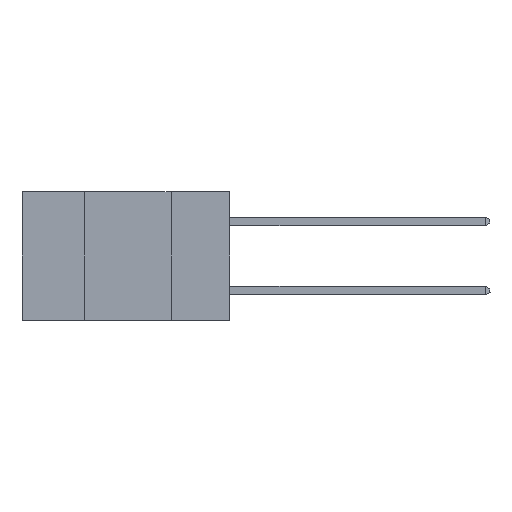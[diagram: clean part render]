
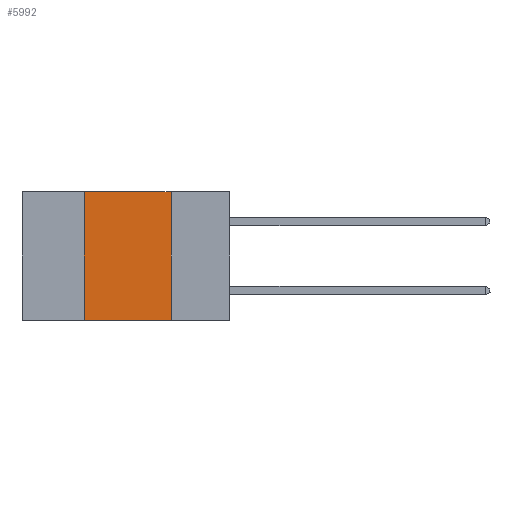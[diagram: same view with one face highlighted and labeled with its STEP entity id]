
A CAD part, left-side view. The second image highlights one B-rep face of the part: STEP entity #5992.
In plain terms, the highlighted planar face has unit normal (-1, 0, 0).
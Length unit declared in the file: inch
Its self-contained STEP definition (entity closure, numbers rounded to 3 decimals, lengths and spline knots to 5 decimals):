
#988 = CARTESIAN_POINT ( 'NONE',  ( 0., 0.6, 0. ) ) ;
#1178 = VERTEX_POINT ( 'NONE', #13964 ) ;
#1229 = VERTEX_POINT ( 'NONE', #21943 ) ;
#1454 = VERTEX_POINT ( 'NONE', #7531 ) ;
#2304 = VERTEX_POINT ( 'NONE', #19432 ) ;
#2470 = ORIENTED_EDGE ( 'NONE', *, *, #5583, .F. ) ;
#2611 = DIRECTION ( 'NONE',  ( 0., -1., 0. ) ) ;
#3014 = DIRECTION ( 'NONE',  ( 0., 0., -1. ) ) ;
#3277 = LINE ( 'NONE', #21633, #22153 ) ;
#3328 = LINE ( 'NONE', #25125, #10076 ) ;
#4059 = EDGE_CURVE ( 'NONE', #1229, #1454, #25564, .T. ) ;
#5583 = EDGE_CURVE ( 'NONE', #1178, #1229, #19972, .T. ) ;
#5795 = CARTESIAN_POINT ( 'NONE',  ( 0., 0.6, 0. ) ) ;
#5992 = ADVANCED_FACE ( 'NONE', ( #25152 ), #9220, .F. ) ;
#6368 = EDGE_CURVE ( 'NONE', #1178, #2304, #3328, .T. ) ;
#7131 = DIRECTION ( 'NONE',  ( 0., 0., -1. ) ) ;
#7194 = EDGE_CURVE ( 'NONE', #1454, #2304, #3277, .T. ) ;
#7531 = CARTESIAN_POINT ( 'NONE',  ( 0., 0.17, 0. ) ) ;
#9220 = PLANE ( 'NONE',  #25579 ) ;
#10076 = VECTOR ( 'NONE', #2611, 39.37008 ) ;
#11253 = DIRECTION ( 'NONE',  ( 1., 0., 0. ) ) ;
#12224 = ORIENTED_EDGE ( 'NONE', *, *, #4059, .F. ) ;
#13964 = CARTESIAN_POINT ( 'NONE',  ( 0., 0.42, -0.37 ) ) ;
#13992 = VECTOR ( 'NONE', #15166, 39.37008 ) ;
#14237 = VECTOR ( 'NONE', #15634, 39.37008 ) ;
#15166 = DIRECTION ( 'NONE',  ( 0., -1., 0. ) ) ;
#15634 = DIRECTION ( 'NONE',  ( 0., 0., 1. ) ) ;
#19432 = CARTESIAN_POINT ( 'NONE',  ( 0., 0.17, -0.37 ) ) ;
#19972 = LINE ( 'NONE', #25878, #14237 ) ;
#20201 = ORIENTED_EDGE ( 'NONE', *, *, #6368, .T. ) ;
#21633 = CARTESIAN_POINT ( 'NONE',  ( 0., 0.17, 0. ) ) ;
#21943 = CARTESIAN_POINT ( 'NONE',  ( 0., 0.42, 0. ) ) ;
#22153 = VECTOR ( 'NONE', #3014, 39.37008 ) ;
#23100 = EDGE_LOOP ( 'NONE', ( #24566, #12224, #2470, #20201 ) ) ;
#24566 = ORIENTED_EDGE ( 'NONE', *, *, #7194, .F. ) ;
#25125 = CARTESIAN_POINT ( 'NONE',  ( 0., 0.6, -0.37 ) ) ;
#25152 = FACE_OUTER_BOUND ( 'NONE', #23100, .T. ) ;
#25564 = LINE ( 'NONE', #5795, #13992 ) ;
#25579 = AXIS2_PLACEMENT_3D ( 'NONE', #988, #11253, #7131 ) ;
#25878 = CARTESIAN_POINT ( 'NONE',  ( 0., 0.42, 0. ) ) ;
